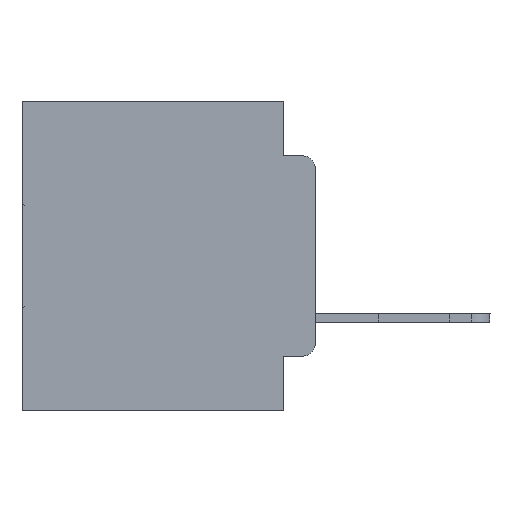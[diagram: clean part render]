
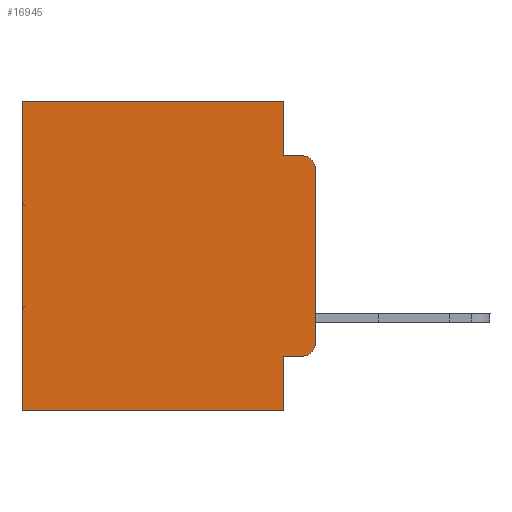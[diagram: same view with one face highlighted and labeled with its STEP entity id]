
A CAD part, left-side view. The second image highlights one B-rep face of the part: STEP entity #16945.
In plain terms, the highlighted planar face has unit normal (-1, 0, 0).
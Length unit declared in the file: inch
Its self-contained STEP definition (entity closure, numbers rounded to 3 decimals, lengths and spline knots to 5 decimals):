
#717 = LINE ( 'NONE', #27624, #19492 ) ;
#764 = VERTEX_POINT ( 'NONE', #28194 ) ;
#1311 = VECTOR ( 'NONE', #23075, 39.37008 ) ;
#1998 = EDGE_LOOP ( 'NONE', ( #26304, #2641, #10727, #19841, #19782, #31587, #5181, #15740, #15709, #25060 ) ) ;
#2065 = DIRECTION ( 'NONE',  ( -1., 0., 0. ) ) ;
#2126 = CARTESIAN_POINT ( 'NONE',  ( 0.298, 0.02, -0.4115 ) ) ;
#2641 = ORIENTED_EDGE ( 'NONE', *, *, #21771, .T. ) ;
#2653 = VERTEX_POINT ( 'NONE', #23271 ) ;
#2753 = LINE ( 'NONE', #5656, #9346 ) ;
#4385 = VERTEX_POINT ( 'NONE', #5162 ) ;
#5162 = CARTESIAN_POINT ( 'NONE',  ( 0.298, 0.051, -0.5 ) ) ;
#5175 = VECTOR ( 'NONE', #6972, 39.37008 ) ;
#5181 = ORIENTED_EDGE ( 'NONE', *, *, #30083, .F. ) ;
#5553 = EDGE_CURVE ( 'NONE', #22513, #4385, #11718, .T. ) ;
#5656 = CARTESIAN_POINT ( 'NONE',  ( 0.298, 0.473, 0. ) ) ;
#5704 = CIRCLE ( 'NONE', #14507, 0.02 ) ;
#6000 = CARTESIAN_POINT ( 'NONE',  ( 0.298, 0.02, -0.1085 ) ) ;
#6632 = EDGE_CURVE ( 'NONE', #22513, #26836, #717, .T. ) ;
#6972 = DIRECTION ( 'NONE',  ( 0., 1., 0. ) ) ;
#7469 = CARTESIAN_POINT ( 'NONE',  ( 0.298, 0.051, 0. ) ) ;
#8205 = CARTESIAN_POINT ( 'NONE',  ( 0.298, 0., 0. ) ) ;
#8751 = VECTOR ( 'NONE', #31659, 39.37008 ) ;
#9331 = CARTESIAN_POINT ( 'NONE',  ( 0.298, 0., -0.5 ) ) ;
#9346 = VECTOR ( 'NONE', #12632, 39.37008 ) ;
#9394 = LINE ( 'NONE', #24445, #5175 ) ;
#10727 = ORIENTED_EDGE ( 'NONE', *, *, #17109, .F. ) ;
#10758 = DIRECTION ( 'NONE',  ( 0., -1., 0. ) ) ;
#10781 = VERTEX_POINT ( 'NONE', #13074 ) ;
#10799 = AXIS2_PLACEMENT_3D ( 'NONE', #14151, #13838, #30865 ) ;
#10969 = VERTEX_POINT ( 'NONE', #31055 ) ;
#11332 = EDGE_CURVE ( 'NONE', #764, #10969, #17596, .T. ) ;
#11718 = LINE ( 'NONE', #19318, #24881 ) ;
#11870 = CARTESIAN_POINT ( 'NONE',  ( 0.298, 0.473, -0.5 ) ) ;
#12206 = AXIS2_PLACEMENT_3D ( 'NONE', #6000, #2065, #20732 ) ;
#12216 = DIRECTION ( 'NONE',  ( -1., 0., 0. ) ) ;
#12632 = DIRECTION ( 'NONE',  ( 0., 0., -1. ) ) ;
#13074 = CARTESIAN_POINT ( 'NONE',  ( 0.298, 0.02, -0.0885 ) ) ;
#13344 = CARTESIAN_POINT ( 'NONE',  ( 0.298, 0.051, -0.4115 ) ) ;
#13522 = CARTESIAN_POINT ( 'NONE',  ( 0.298, 0.02, -0.3915 ) ) ;
#13838 = DIRECTION ( 'NONE',  ( 1., 0., 0. ) ) ;
#14151 = CARTESIAN_POINT ( 'NONE',  ( 0.298, 0., 0. ) ) ;
#14507 = AXIS2_PLACEMENT_3D ( 'NONE', #13522, #12216, #14805 ) ;
#14598 = VECTOR ( 'NONE', #18921, 39.37008 ) ;
#14805 = DIRECTION ( 'NONE',  ( 0., 0., -1. ) ) ;
#15709 = ORIENTED_EDGE ( 'NONE', *, *, #6632, .T. ) ;
#15740 = ORIENTED_EDGE ( 'NONE', *, *, #5553, .F. ) ;
#16161 = VECTOR ( 'NONE', #28781, 39.37008 ) ;
#16945 = ADVANCED_FACE ( 'NONE', ( #23861 ), #31340, .F. ) ;
#17061 = CARTESIAN_POINT ( 'NONE',  ( 0.298, 0.051, -0.0885 ) ) ;
#17109 = EDGE_CURVE ( 'NONE', #18233, #10781, #21742, .T. ) ;
#17596 = LINE ( 'NONE', #8205, #1311 ) ;
#18233 = VERTEX_POINT ( 'NONE', #26306 ) ;
#18304 = EDGE_CURVE ( 'NONE', #26836, #10969, #5704, .T. ) ;
#18921 = DIRECTION ( 'NONE',  ( 0., 0., -1. ) ) ;
#19318 = CARTESIAN_POINT ( 'NONE',  ( 0.298, 0.051, 0. ) ) ;
#19492 = VECTOR ( 'NONE', #10758, 39.37008 ) ;
#19782 = ORIENTED_EDGE ( 'NONE', *, *, #27949, .T. ) ;
#19841 = ORIENTED_EDGE ( 'NONE', *, *, #29720, .F. ) ;
#20732 = DIRECTION ( 'NONE',  ( 0., 0., -1. ) ) ;
#21742 = LINE ( 'NONE', #17061, #8751 ) ;
#21771 = EDGE_CURVE ( 'NONE', #764, #10781, #25109, .T. ) ;
#22513 = VERTEX_POINT ( 'NONE', #13344 ) ;
#22876 = VERTEX_POINT ( 'NONE', #11870 ) ;
#23075 = DIRECTION ( 'NONE',  ( 0., 0., -1. ) ) ;
#23271 = CARTESIAN_POINT ( 'NONE',  ( 0.298, 0.473, 0. ) ) ;
#23774 = LINE ( 'NONE', #31245, #14598 ) ;
#23861 = FACE_OUTER_BOUND ( 'NONE', #1998, .T. ) ;
#24056 = LINE ( 'NONE', #9331, #16161 ) ;
#24445 = CARTESIAN_POINT ( 'NONE',  ( 0.298, 0., 0. ) ) ;
#24881 = VECTOR ( 'NONE', #29394, 39.37008 ) ;
#25060 = ORIENTED_EDGE ( 'NONE', *, *, #18304, .T. ) ;
#25109 = CIRCLE ( 'NONE', #12206, 0.02 ) ;
#26304 = ORIENTED_EDGE ( 'NONE', *, *, #11332, .F. ) ;
#26306 = CARTESIAN_POINT ( 'NONE',  ( 0.298, 0.051, -0.0885 ) ) ;
#26836 = VERTEX_POINT ( 'NONE', #2126 ) ;
#26990 = EDGE_CURVE ( 'NONE', #2653, #22876, #2753, .T. ) ;
#27043 = VERTEX_POINT ( 'NONE', #7469 ) ;
#27624 = CARTESIAN_POINT ( 'NONE',  ( 0.298, 0.051, -0.4115 ) ) ;
#27949 = EDGE_CURVE ( 'NONE', #27043, #2653, #9394, .T. ) ;
#28194 = CARTESIAN_POINT ( 'NONE',  ( 0.298, 0., -0.1085 ) ) ;
#28781 = DIRECTION ( 'NONE',  ( 0., 1., 0. ) ) ;
#29394 = DIRECTION ( 'NONE',  ( 0., 0., -1. ) ) ;
#29720 = EDGE_CURVE ( 'NONE', #27043, #18233, #23774, .T. ) ;
#30083 = EDGE_CURVE ( 'NONE', #4385, #22876, #24056, .T. ) ;
#30865 = DIRECTION ( 'NONE',  ( 0., 0., -1. ) ) ;
#31055 = CARTESIAN_POINT ( 'NONE',  ( 0.298, 0., -0.3915 ) ) ;
#31245 = CARTESIAN_POINT ( 'NONE',  ( 0.298, 0.051, 0. ) ) ;
#31340 = PLANE ( 'NONE',  #10799 ) ;
#31587 = ORIENTED_EDGE ( 'NONE', *, *, #26990, .T. ) ;
#31659 = DIRECTION ( 'NONE',  ( 0., -1., 0. ) ) ;
